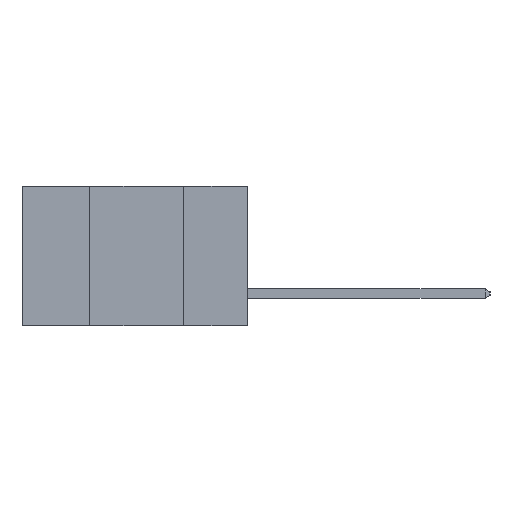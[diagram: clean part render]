
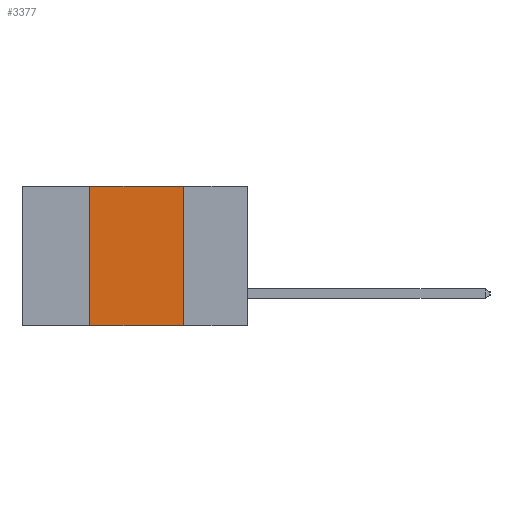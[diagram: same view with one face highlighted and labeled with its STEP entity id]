
A CAD part, left-side view. The second image highlights one B-rep face of the part: STEP entity #3377.
In plain terms, the highlighted planar face has unit normal (-1, 0, 0).
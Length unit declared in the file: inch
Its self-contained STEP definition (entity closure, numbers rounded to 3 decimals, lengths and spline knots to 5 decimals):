
#691 = LINE ( 'NONE', #10357, #3690 ) ;
#710 = DIRECTION ( 'NONE',  ( 0., 0., 1. ) ) ;
#1023 = LINE ( 'NONE', #6762, #4327 ) ;
#1251 = VECTOR ( 'NONE', #12032, 39.37008 ) ;
#1498 = CARTESIAN_POINT ( 'NONE',  ( 0., 0.17, -0.37 ) ) ;
#2439 = CARTESIAN_POINT ( 'NONE',  ( 0., 0.42, 0. ) ) ;
#2616 = VERTEX_POINT ( 'NONE', #10672 ) ;
#3377 = ADVANCED_FACE ( 'NONE', ( #6178 ), #11098, .F. ) ;
#3690 = VECTOR ( 'NONE', #13376, 39.37008 ) ;
#4056 = EDGE_CURVE ( 'NONE', #2616, #11647, #12949, .T. ) ;
#4327 = VECTOR ( 'NONE', #710, 39.37008 ) ;
#5370 = VECTOR ( 'NONE', #6941, 39.37008 ) ;
#5663 = CARTESIAN_POINT ( 'NONE',  ( 0., 0.6, 0. ) ) ;
#6178 = FACE_OUTER_BOUND ( 'NONE', #6691, .T. ) ;
#6464 = ORIENTED_EDGE ( 'NONE', *, *, #8987, .F. ) ;
#6636 = EDGE_CURVE ( 'NONE', #2616, #13187, #1023, .T. ) ;
#6691 = EDGE_LOOP ( 'NONE', ( #6464, #12518, #9346, #9054 ) ) ;
#6746 = AXIS2_PLACEMENT_3D ( 'NONE', #5663, #7980, #11007 ) ;
#6762 = CARTESIAN_POINT ( 'NONE',  ( 0., 0.42, -0.37 ) ) ;
#6941 = DIRECTION ( 'NONE',  ( 0., 0., -1. ) ) ;
#6950 = VERTEX_POINT ( 'NONE', #9113 ) ;
#7446 = CARTESIAN_POINT ( 'NONE',  ( 0., 0.17, -0.37 ) ) ;
#7980 = DIRECTION ( 'NONE',  ( 1., 0., 0. ) ) ;
#8987 = EDGE_CURVE ( 'NONE', #6950, #11647, #11080, .T. ) ;
#9054 = ORIENTED_EDGE ( 'NONE', *, *, #4056, .T. ) ;
#9113 = CARTESIAN_POINT ( 'NONE',  ( 0., 0.17, 0. ) ) ;
#9346 = ORIENTED_EDGE ( 'NONE', *, *, #6636, .F. ) ;
#10357 = CARTESIAN_POINT ( 'NONE',  ( 0., 0.6, 0. ) ) ;
#10672 = CARTESIAN_POINT ( 'NONE',  ( 0., 0.42, -0.37 ) ) ;
#10726 = EDGE_CURVE ( 'NONE', #13187, #6950, #691, .T. ) ;
#10902 = CARTESIAN_POINT ( 'NONE',  ( 0., 0.6, -0.37 ) ) ;
#11007 = DIRECTION ( 'NONE',  ( 0., 0., -1. ) ) ;
#11080 = LINE ( 'NONE', #1498, #5370 ) ;
#11098 = PLANE ( 'NONE',  #6746 ) ;
#11647 = VERTEX_POINT ( 'NONE', #7446 ) ;
#12032 = DIRECTION ( 'NONE',  ( 0., -1., 0. ) ) ;
#12518 = ORIENTED_EDGE ( 'NONE', *, *, #10726, .F. ) ;
#12949 = LINE ( 'NONE', #10902, #1251 ) ;
#13187 = VERTEX_POINT ( 'NONE', #2439 ) ;
#13376 = DIRECTION ( 'NONE',  ( 0., -1., 0. ) ) ;
